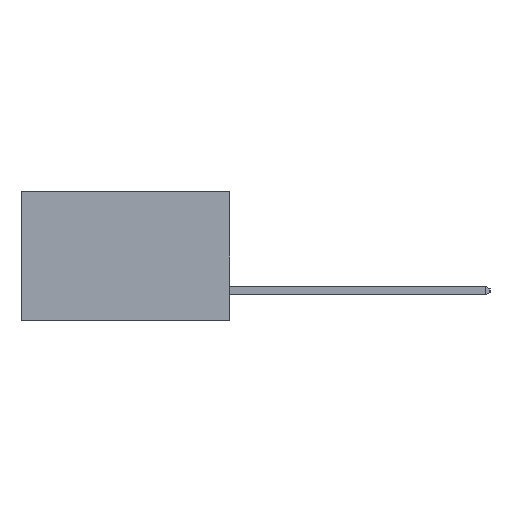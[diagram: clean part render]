
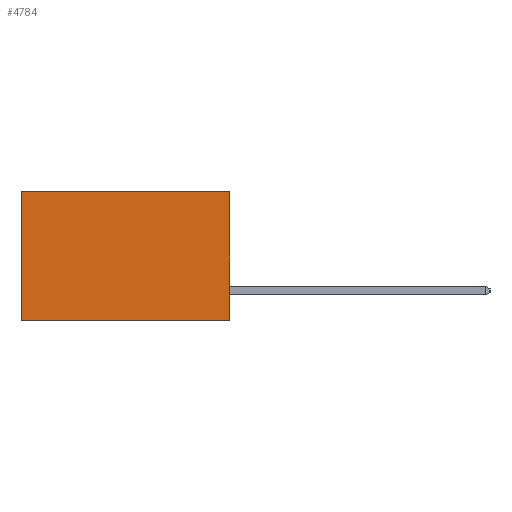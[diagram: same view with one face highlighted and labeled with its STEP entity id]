
A CAD part, left-side view. The second image highlights one B-rep face of the part: STEP entity #4784.
In plain terms, the highlighted planar face has unit normal (-1, 0, 0).
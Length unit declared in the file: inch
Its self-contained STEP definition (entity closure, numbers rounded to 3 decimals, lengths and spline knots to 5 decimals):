
#193 = DIRECTION ( 'NONE',  ( 0., 1., 0. ) ) ;
#230 = CARTESIAN_POINT ( 'NONE',  ( 0.2615, 0., -0.37 ) ) ;
#255 = VERTEX_POINT ( 'NONE', #7049 ) ;
#616 = DIRECTION ( 'NONE',  ( 0., 1., 0. ) ) ;
#1875 = LINE ( 'NONE', #9300, #11380 ) ;
#2020 = VECTOR ( 'NONE', #10597, 39.37008 ) ;
#2082 = EDGE_CURVE ( 'NONE', #15240, #8878, #9028, .T. ) ;
#2127 = FACE_OUTER_BOUND ( 'NONE', #2148, .T. ) ;
#2148 = EDGE_LOOP ( 'NONE', ( #8029, #4762, #9722, #11137 ) ) ;
#2313 = EDGE_CURVE ( 'NONE', #8621, #255, #12255, .T. ) ;
#2642 = DIRECTION ( 'NONE',  ( 0., 0., -1. ) ) ;
#2676 = CARTESIAN_POINT ( 'NONE',  ( 0.2615, 0.6, -0.37 ) ) ;
#4762 = ORIENTED_EDGE ( 'NONE', *, *, #5903, .F. ) ;
#4784 = ADVANCED_FACE ( 'NONE', ( #2127 ), #13817, .F. ) ;
#4814 = VECTOR ( 'NONE', #193, 39.37008 ) ;
#5903 = EDGE_CURVE ( 'NONE', #255, #8878, #14564, .T. ) ;
#6398 = EDGE_CURVE ( 'NONE', #8621, #15240, #1875, .T. ) ;
#7049 = CARTESIAN_POINT ( 'NONE',  ( 0.2615, 0., -0.37 ) ) ;
#7132 = AXIS2_PLACEMENT_3D ( 'NONE', #14025, #13783, #13765 ) ;
#8029 = ORIENTED_EDGE ( 'NONE', *, *, #2082, .T. ) ;
#8621 = VERTEX_POINT ( 'NONE', #14125 ) ;
#8878 = VERTEX_POINT ( 'NONE', #10232 ) ;
#9028 = LINE ( 'NONE', #2676, #12620 ) ;
#9300 = CARTESIAN_POINT ( 'NONE',  ( 0.2615, 0., 0. ) ) ;
#9722 = ORIENTED_EDGE ( 'NONE', *, *, #2313, .F. ) ;
#10232 = CARTESIAN_POINT ( 'NONE',  ( 0.2615, 0.6, -0.37 ) ) ;
#10251 = CARTESIAN_POINT ( 'NONE',  ( 0.2615, 0.6, 0. ) ) ;
#10597 = DIRECTION ( 'NONE',  ( 0., 0., -1. ) ) ;
#11137 = ORIENTED_EDGE ( 'NONE', *, *, #6398, .T. ) ;
#11380 = VECTOR ( 'NONE', #616, 39.37008 ) ;
#12255 = LINE ( 'NONE', #15067, #2020 ) ;
#12620 = VECTOR ( 'NONE', #2642, 39.37008 ) ;
#13765 = DIRECTION ( 'NONE',  ( 0., 0., -1. ) ) ;
#13783 = DIRECTION ( 'NONE',  ( 1., 0., 0. ) ) ;
#13817 = PLANE ( 'NONE',  #7132 ) ;
#14025 = CARTESIAN_POINT ( 'NONE',  ( 0.2615, 0., -0.37 ) ) ;
#14125 = CARTESIAN_POINT ( 'NONE',  ( 0.2615, 0., 0. ) ) ;
#14564 = LINE ( 'NONE', #230, #4814 ) ;
#15067 = CARTESIAN_POINT ( 'NONE',  ( 0.2615, 0., -0.37 ) ) ;
#15240 = VERTEX_POINT ( 'NONE', #10251 ) ;
